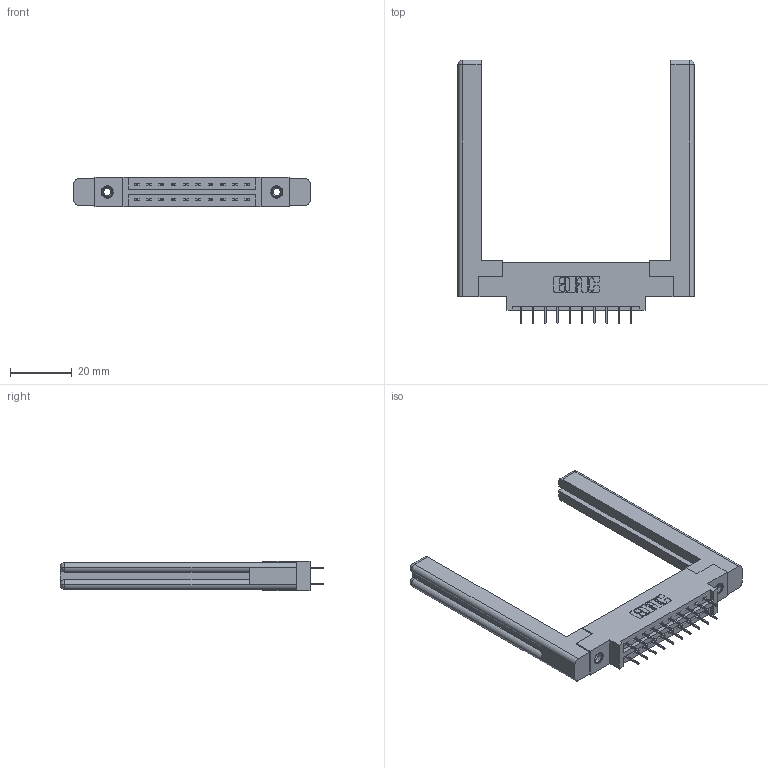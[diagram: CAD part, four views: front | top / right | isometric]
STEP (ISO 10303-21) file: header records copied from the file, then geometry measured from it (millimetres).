
FILE_DESCRIPTION (( 'STEP AP203' ), '1' );
FILE_NAME ('387-020-524-858.STEP', '2019-10-16T15:21:14', ( '' ), ( '' ), 'SwSTEP 2.0', 'SolidWorks 2016', '' );
FILE_SCHEMA (( 'CONFIG_CONTROL_DESIGN' ));
Length unit declared in the file: inch
Products named in the file (5): 345-250-001_345-250-001-102; 307-220-058; 387-020-524-858; 345-292-001_345-293-124; 337 Part_0.170 Offset - 0.156 Dia-TI
Assembly tree (25 placements, depth 2):
  387-020-524-858
    337 Part_0.170 Offset - 0.156 Dia-TI
    345-292-001_345-293-124  x20
    345-250-001_345-250-001-102  x2
    307-220-058  x2
Bounding box: 76.25 x 85.1 x 9.4 mm (x, y, z)
Volume: 14604.5 mm3; surface area: 13186 mm2
Topology: 25 solids, 25 shells, 1420 faces, 3977 edges, 2558 vertices
Faces by surface type: plane 1038, cylinder 358, cone 12, torus 12
Entity records: 14732 total; most frequent: CARTESIAN_POINT 2517, ORIENTED_EDGE 2392, DIRECTION 2216, EDGE_CURVE 1196, LINE 1024, VECTOR 1024, VERTEX_POINT 786, AXIS2_PLACEMENT_3D 596
